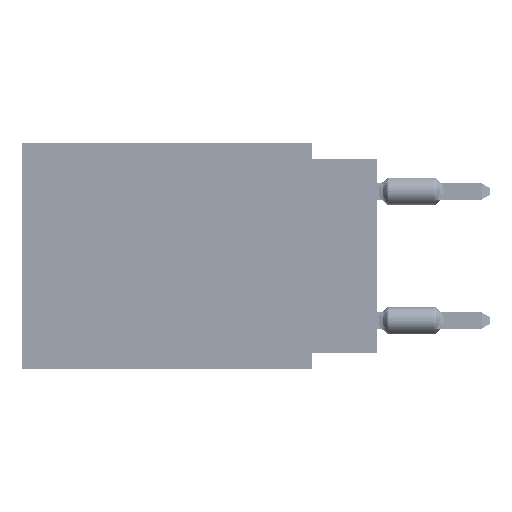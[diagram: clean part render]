
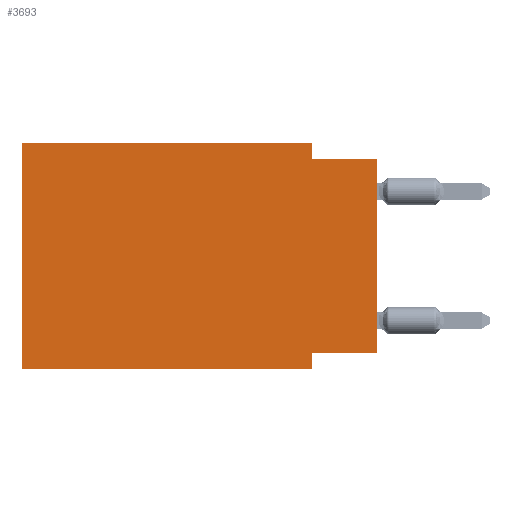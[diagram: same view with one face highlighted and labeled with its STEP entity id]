
A CAD part, left-side view. The second image highlights one B-rep face of the part: STEP entity #3693.
In plain terms, the highlighted planar face has unit normal (-1, 0, 0).
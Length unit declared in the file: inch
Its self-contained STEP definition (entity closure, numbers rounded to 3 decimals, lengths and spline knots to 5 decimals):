
#2208 = PLANE ( 'NONE',  #65978 ) ;
#2717 = LINE ( 'NONE', #8142, #20747 ) ;
#3693 = ADVANCED_FACE ( 'NONE', ( #18392 ), #2208, .F. ) ;
#4545 = CARTESIAN_POINT ( 'NONE',  ( 0., 0.1, -0.325 ) ) ;
#5278 = CARTESIAN_POINT ( 'NONE',  ( 0., 0.1, -0.025 ) ) ;
#5721 = ORIENTED_EDGE ( 'NONE', *, *, #87630, .F. ) ;
#7106 = CARTESIAN_POINT ( 'NONE',  ( 0., 0.1, 0. ) ) ;
#7149 = VERTEX_POINT ( 'NONE', #5278 ) ;
#8142 = CARTESIAN_POINT ( 'NONE',  ( 0., 0.55, -0.35 ) ) ;
#9049 = CARTESIAN_POINT ( 'NONE',  ( 0., 0.55, 0. ) ) ;
#9628 = CARTESIAN_POINT ( 'NONE',  ( 0., 0.55, -0.35 ) ) ;
#12801 = VECTOR ( 'NONE', #26538, 39.37008 ) ;
#15663 = LINE ( 'NONE', #66916, #85461 ) ;
#15851 = DIRECTION ( 'NONE',  ( 1., 0., 0. ) ) ;
#16853 = CARTESIAN_POINT ( 'NONE',  ( 0., 0.55, 0. ) ) ;
#17052 = VECTOR ( 'NONE', #19874, 39.37008 ) ;
#18392 = FACE_OUTER_BOUND ( 'NONE', #74664, .T. ) ;
#19259 = EDGE_CURVE ( 'NONE', #36370, #51873, #15663, .T. ) ;
#19874 = DIRECTION ( 'NONE',  ( 0., 0., 1. ) ) ;
#20747 = VECTOR ( 'NONE', #48649, 39.37008 ) ;
#23072 = ORIENTED_EDGE ( 'NONE', *, *, #19259, .F. ) ;
#25314 = CARTESIAN_POINT ( 'NONE',  ( 0., 0.1, -0.35 ) ) ;
#26538 = DIRECTION ( 'NONE',  ( 0., 0., 1. ) ) ;
#31237 = VERTEX_POINT ( 'NONE', #45645 ) ;
#32333 = DIRECTION ( 'NONE',  ( 0., -1., 0. ) ) ;
#33517 = EDGE_CURVE ( 'NONE', #51873, #80979, #81278, .T. ) ;
#34892 = ORIENTED_EDGE ( 'NONE', *, *, #74126, .F. ) ;
#35125 = LINE ( 'NONE', #79646, #86979 ) ;
#35454 = EDGE_CURVE ( 'NONE', #63657, #80979, #2717, .T. ) ;
#35730 = CARTESIAN_POINT ( 'NONE',  ( 0., 0.1, -0.35 ) ) ;
#36370 = VERTEX_POINT ( 'NONE', #44641 ) ;
#38894 = DIRECTION ( 'NONE',  ( 0., 0., -1. ) ) ;
#40201 = CARTESIAN_POINT ( 'NONE',  ( 0., 0.1, 0. ) ) ;
#43589 = LINE ( 'NONE', #7106, #79628 ) ;
#44641 = CARTESIAN_POINT ( 'NONE',  ( 0., 0., -0.325 ) ) ;
#45645 = CARTESIAN_POINT ( 'NONE',  ( 0., 0., -0.025 ) ) ;
#46608 = LINE ( 'NONE', #67042, #12801 ) ;
#48649 = DIRECTION ( 'NONE',  ( 0., -1., 0. ) ) ;
#49046 = EDGE_CURVE ( 'NONE', #36370, #31237, #75247, .T. ) ;
#51873 = VERTEX_POINT ( 'NONE', #4545 ) ;
#52425 = CARTESIAN_POINT ( 'NONE',  ( 0., 0.55, 0. ) ) ;
#53543 = CARTESIAN_POINT ( 'NONE',  ( 0., 0., 0. ) ) ;
#54405 = DIRECTION ( 'NONE',  ( 0., 0., -1. ) ) ;
#56117 = ORIENTED_EDGE ( 'NONE', *, *, #60569, .F. ) ;
#57367 = ORIENTED_EDGE ( 'NONE', *, *, #33517, .F. ) ;
#60569 = EDGE_CURVE ( 'NONE', #7149, #31237, #35125, .T. ) ;
#61122 = VECTOR ( 'NONE', #32333, 39.37008 ) ;
#63134 = DIRECTION ( 'NONE',  ( 0., 0., -1. ) ) ;
#63283 = VECTOR ( 'NONE', #38894, 39.37008 ) ;
#63657 = VERTEX_POINT ( 'NONE', #9628 ) ;
#65978 = AXIS2_PLACEMENT_3D ( 'NONE', #9049, #15851, #63134 ) ;
#66625 = DIRECTION ( 'NONE',  ( 0., 1., 0. ) ) ;
#66916 = CARTESIAN_POINT ( 'NONE',  ( 0., 0., -0.325 ) ) ;
#67042 = CARTESIAN_POINT ( 'NONE',  ( 0., 0.55, 0. ) ) ;
#70070 = EDGE_CURVE ( 'NONE', #63657, #86223, #46608, .T. ) ;
#70264 = ORIENTED_EDGE ( 'NONE', *, *, #49046, .T. ) ;
#72951 = VERTEX_POINT ( 'NONE', #40201 ) ;
#74126 = EDGE_CURVE ( 'NONE', #86223, #72951, #79179, .T. ) ;
#74664 = EDGE_LOOP ( 'NONE', ( #70264, #56117, #5721, #34892, #77497, #82277, #57367, #23072 ) ) ;
#75247 = LINE ( 'NONE', #53543, #17052 ) ;
#77497 = ORIENTED_EDGE ( 'NONE', *, *, #70070, .F. ) ;
#79179 = LINE ( 'NONE', #52425, #61122 ) ;
#79628 = VECTOR ( 'NONE', #54405, 39.37008 ) ;
#79646 = CARTESIAN_POINT ( 'NONE',  ( 0., 0., -0.025 ) ) ;
#80979 = VERTEX_POINT ( 'NONE', #35730 ) ;
#81278 = LINE ( 'NONE', #25314, #63283 ) ;
#82277 = ORIENTED_EDGE ( 'NONE', *, *, #35454, .T. ) ;
#85461 = VECTOR ( 'NONE', #66625, 39.37008 ) ;
#86223 = VERTEX_POINT ( 'NONE', #16853 ) ;
#86408 = DIRECTION ( 'NONE',  ( 0., -1., 0. ) ) ;
#86979 = VECTOR ( 'NONE', #86408, 39.37008 ) ;
#87630 = EDGE_CURVE ( 'NONE', #72951, #7149, #43589, .T. ) ;
